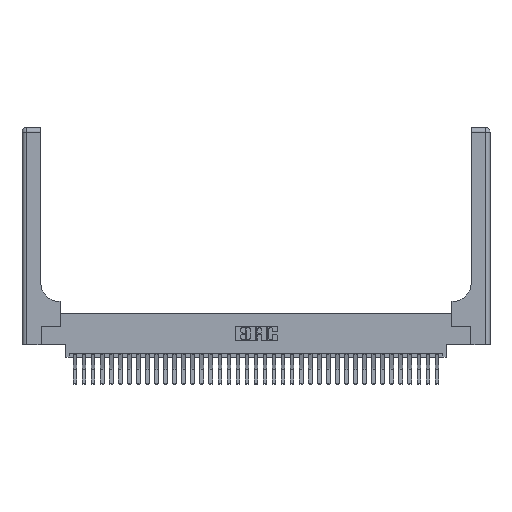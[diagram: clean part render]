
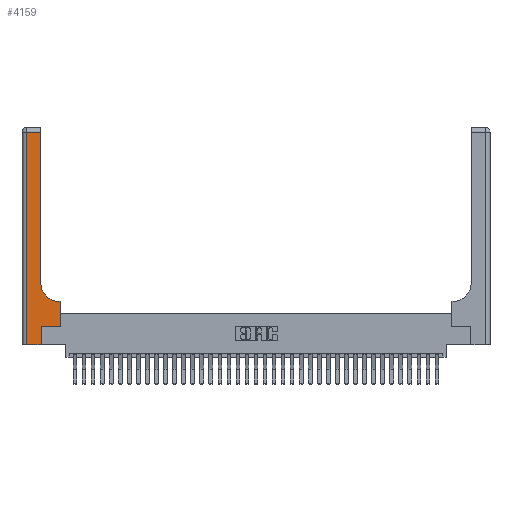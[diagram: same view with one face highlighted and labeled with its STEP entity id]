
A CAD part, top view. The second image highlights one B-rep face of the part: STEP entity #4159.
In plain terms, the highlighted planar face has unit normal (0, 0, 1).
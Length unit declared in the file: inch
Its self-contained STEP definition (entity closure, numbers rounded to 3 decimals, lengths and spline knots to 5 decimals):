
#774 = DIRECTION ( 'NONE',  ( 0., 0., -1. ) ) ;
#1165 = CARTESIAN_POINT ( 'NONE',  ( 0.528, 0.25, 0.37 ) ) ;
#1414 = CARTESIAN_POINT ( 'NONE',  ( 0.26, 3., 0.37 ) ) ;
#1657 = DIRECTION ( 'NONE',  ( 0., -1., 0. ) ) ;
#1963 = LINE ( 'NONE', #9582, #2936 ) ;
#1967 = EDGE_CURVE ( 'NONE', #10175, #4450, #28858, .T. ) ;
#2084 = EDGE_CURVE ( 'NONE', #22970, #30496, #22027, .T. ) ;
#2516 = VERTEX_POINT ( 'NONE', #16716 ) ;
#2936 = VECTOR ( 'NONE', #4605, 39.37008 ) ;
#3577 = DIRECTION ( 'NONE',  ( -1., 0., 0. ) ) ;
#3725 = VERTEX_POINT ( 'NONE', #20702 ) ;
#4018 = ORIENTED_EDGE ( 'NONE', *, *, #1967, .T. ) ;
#4159 = ADVANCED_FACE ( 'NONE', ( #10718 ), #18354, .F. ) ;
#4450 = VERTEX_POINT ( 'NONE', #23113 ) ;
#4605 = DIRECTION ( 'NONE',  ( 1., 0., 0. ) ) ;
#5665 = CARTESIAN_POINT ( 'NONE',  ( 0.26, 0.6, 0.37 ) ) ;
#5997 = EDGE_CURVE ( 'NONE', #29480, #3725, #11570, .T. ) ;
#6245 = VECTOR ( 'NONE', #29053, 39.37008 ) ;
#6863 = LINE ( 'NONE', #1414, #12075 ) ;
#6902 = CARTESIAN_POINT ( 'NONE',  ( 0., 2.94, 0.37 ) ) ;
#7243 = ORIENTED_EDGE ( 'NONE', *, *, #25957, .T. ) ;
#7707 = EDGE_CURVE ( 'NONE', #25116, #2516, #11312, .T. ) ;
#8016 = EDGE_LOOP ( 'NONE', ( #25765, #7243, #22314, #22595, #31025, #10746, #4018, #13232, #8931 ) ) ;
#8276 = VECTOR ( 'NONE', #29536, 39.37008 ) ;
#8402 = AXIS2_PLACEMENT_3D ( 'NONE', #23481, #774, #3577 ) ;
#8931 = ORIENTED_EDGE ( 'NONE', *, *, #5997, .T. ) ;
#9311 = CARTESIAN_POINT ( 'NONE',  ( 0.265, 0.25, 0.37 ) ) ;
#9582 = CARTESIAN_POINT ( 'NONE',  ( 0., 0., 0.37 ) ) ;
#10083 = CARTESIAN_POINT ( 'NONE',  ( 0.06, 0., 0.37 ) ) ;
#10175 = VERTEX_POINT ( 'NONE', #20844 ) ;
#10718 = FACE_OUTER_BOUND ( 'NONE', #8016, .T. ) ;
#10746 = ORIENTED_EDGE ( 'NONE', *, *, #23106, .T. ) ;
#11312 = LINE ( 'NONE', #18778, #6245 ) ;
#11570 = CIRCLE ( 'NONE', #12045, 0.25 ) ;
#11577 = LINE ( 'NONE', #6902, #26421 ) ;
#12045 = AXIS2_PLACEMENT_3D ( 'NONE', #25621, #28269, #18497 ) ;
#12075 = VECTOR ( 'NONE', #27111, 39.37008 ) ;
#13232 = ORIENTED_EDGE ( 'NONE', *, *, #29456, .T. ) ;
#14196 = VECTOR ( 'NONE', #1657, 39.37008 ) ;
#15789 = DIRECTION ( 'NONE',  ( -1., 0., 0. ) ) ;
#16716 = CARTESIAN_POINT ( 'NONE',  ( 0.265, 0.25, 0.37 ) ) ;
#17838 = EDGE_CURVE ( 'NONE', #30496, #25116, #1963, .T. ) ;
#18354 = PLANE ( 'NONE',  #8402 ) ;
#18425 = DIRECTION ( 'NONE',  ( 0., 1., 0. ) ) ;
#18497 = DIRECTION ( 'NONE',  ( 1., 0., 0. ) ) ;
#18778 = CARTESIAN_POINT ( 'NONE',  ( 0.265, 0., 0.37 ) ) ;
#19188 = DIRECTION ( 'NONE',  ( -1., 0., 0. ) ) ;
#19409 = CARTESIAN_POINT ( 'NONE',  ( 0.51, 0.6, 0.37 ) ) ;
#20171 = VECTOR ( 'NONE', #18425, 39.37008 ) ;
#20702 = CARTESIAN_POINT ( 'NONE',  ( 0.26, 0.85, 0.37 ) ) ;
#20844 = CARTESIAN_POINT ( 'NONE',  ( 0.528, 0.25, 0.37 ) ) ;
#21029 = VERTEX_POINT ( 'NONE', #26981 ) ;
#22027 = LINE ( 'NONE', #29017, #14196 ) ;
#22314 = ORIENTED_EDGE ( 'NONE', *, *, #2084, .T. ) ;
#22595 = ORIENTED_EDGE ( 'NONE', *, *, #17838, .T. ) ;
#22970 = VERTEX_POINT ( 'NONE', #24416 ) ;
#23106 = EDGE_CURVE ( 'NONE', #2516, #10175, #32030, .T. ) ;
#23113 = CARTESIAN_POINT ( 'NONE',  ( 0.528, 0.6, 0.37 ) ) ;
#23481 = CARTESIAN_POINT ( 'NONE',  ( 0., 3., 0.37 ) ) ;
#24416 = CARTESIAN_POINT ( 'NONE',  ( 0.06, 2.94, 0.37 ) ) ;
#25116 = VERTEX_POINT ( 'NONE', #29304 ) ;
#25621 = CARTESIAN_POINT ( 'NONE',  ( 0.51, 0.85, 0.37 ) ) ;
#25736 = LINE ( 'NONE', #5665, #26506 ) ;
#25765 = ORIENTED_EDGE ( 'NONE', *, *, #26415, .T. ) ;
#25957 = EDGE_CURVE ( 'NONE', #21029, #22970, #11577, .T. ) ;
#26415 = EDGE_CURVE ( 'NONE', #3725, #21029, #6863, .T. ) ;
#26421 = VECTOR ( 'NONE', #19188, 39.37008 ) ;
#26506 = VECTOR ( 'NONE', #15789, 39.37008 ) ;
#26981 = CARTESIAN_POINT ( 'NONE',  ( 0.26, 2.94, 0.37 ) ) ;
#27111 = DIRECTION ( 'NONE',  ( 0., 1., 0. ) ) ;
#28269 = DIRECTION ( 'NONE',  ( 0., 0., -1. ) ) ;
#28858 = LINE ( 'NONE', #1165, #20171 ) ;
#29017 = CARTESIAN_POINT ( 'NONE',  ( 0.06, 3., 0.37 ) ) ;
#29053 = DIRECTION ( 'NONE',  ( 0., 1., 0. ) ) ;
#29304 = CARTESIAN_POINT ( 'NONE',  ( 0.265, 0., 0.37 ) ) ;
#29456 = EDGE_CURVE ( 'NONE', #4450, #29480, #25736, .T. ) ;
#29480 = VERTEX_POINT ( 'NONE', #19409 ) ;
#29536 = DIRECTION ( 'NONE',  ( 1., 0., 0. ) ) ;
#30496 = VERTEX_POINT ( 'NONE', #10083 ) ;
#31025 = ORIENTED_EDGE ( 'NONE', *, *, #7707, .T. ) ;
#32030 = LINE ( 'NONE', #9311, #8276 ) ;
